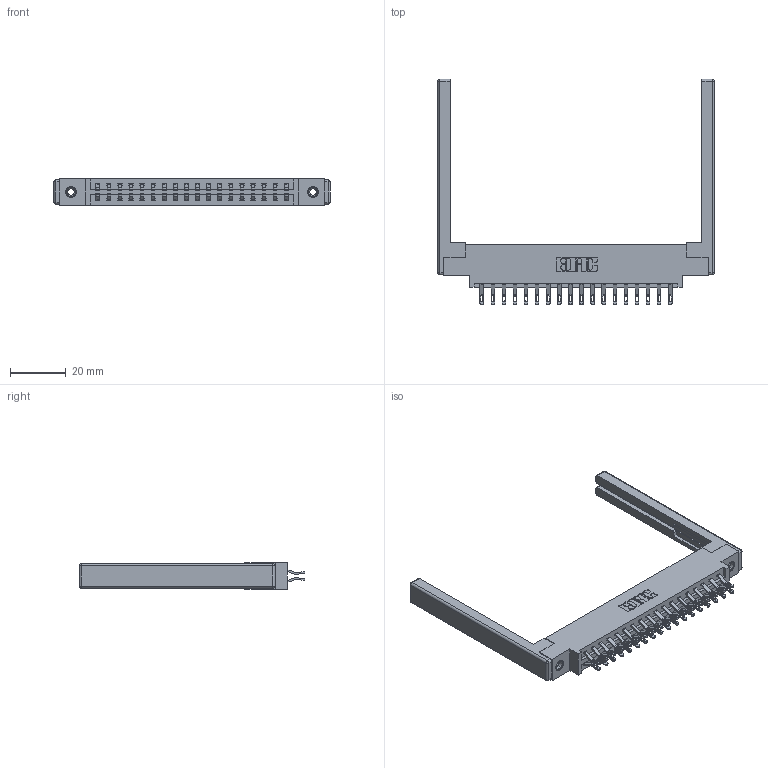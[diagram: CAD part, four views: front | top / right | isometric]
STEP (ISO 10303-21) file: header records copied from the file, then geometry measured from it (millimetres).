
FILE_DESCRIPTION (( 'STEP AP203' ), '1' );
FILE_NAME ('387-036-555-868.STEP', '2019-10-17T19:57:39', ( '' ), ( '' ), 'SwSTEP 2.0', 'SolidWorks 2016', '' );
FILE_SCHEMA (( 'CONFIG_CONTROL_DESIGN' ));
Length unit declared in the file: inch
Products named in the file (5): 345-292-001_555 Tail; 387-036-555-868; 307-220-068; 345-250-001_345-250-001-102; 337 Part_0.170 Offset - 0.156 Dia-TI
Assembly tree (41 placements, depth 2):
  387-036-555-868
    337 Part_0.170 Offset - 0.156 Dia-TI
    345-292-001_555 Tail  x36
    345-250-001_345-250-001-102  x2
    307-220-068  x2
Bounding box: 98.76 x 80.52 x 9.4 mm (x, y, z)
Volume: 14459.8 mm3; surface area: 15692.5 mm2
Topology: 41 solids, 41 shells, 2432 faces, 7517 edges, 4990 vertices
Faces by surface type: plane 1458, cylinder 950, cone 12, sphere 8, torus 4
Entity records: 20278 total; most frequent: CARTESIAN_POINT 3437, ORIENTED_EDGE 3332, DIRECTION 3008, EDGE_CURVE 1666, LINE 1468, VECTOR 1468, VERTEX_POINT 1102, AXIS2_PLACEMENT_3D 770
